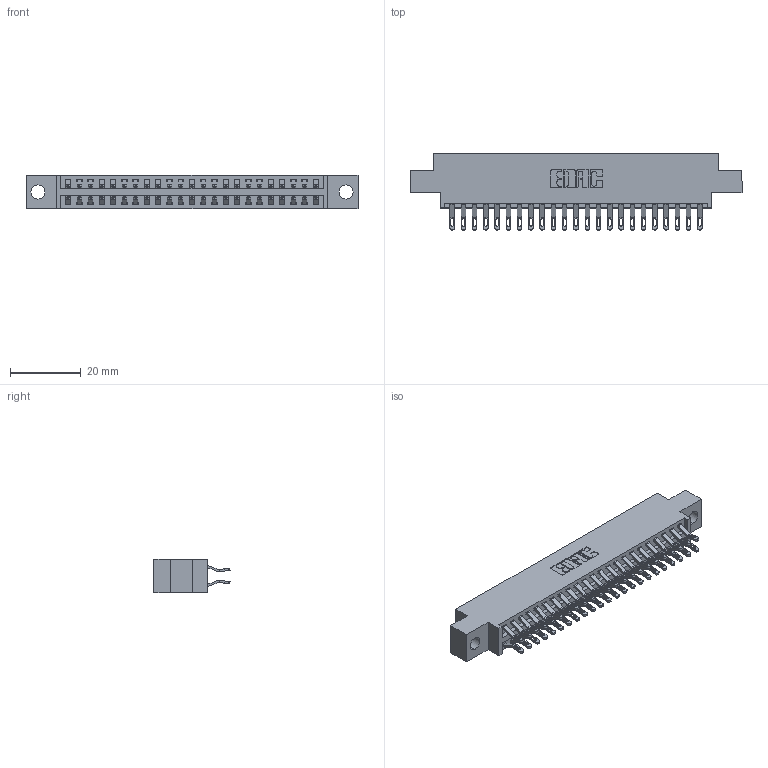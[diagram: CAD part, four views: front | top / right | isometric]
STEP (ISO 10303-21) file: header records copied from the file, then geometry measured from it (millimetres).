
FILE_DESCRIPTION (( 'STEP AP203' ), '1' );
FILE_NAME ('396-046-555-804.STEP', '2018-09-07T09:04:24', ( '' ), ( '' ), 'SwSTEP 2.0', 'SolidWorks 2016', '' );
FILE_SCHEMA (( 'CONFIG_CONTROL_DESIGN' ));
Length unit declared in the file: inch
Products named in the file (3): 346 Part_0.170 Offset - 0.156 Dia-TH; 345-292-001_555 Tail; 396-046-555-804
Assembly tree (47 placements, depth 2):
  396-046-555-804
    346 Part_0.170 Offset - 0.156 Dia-TH
    345-292-001_555 Tail  x46
Bounding box: 93.6 x 21.46 x 9.4 mm (x, y, z)
Volume: 8870.5 mm3; surface area: 12363 mm2
Topology: 47 solids, 47 shells, 2794 faces, 8759 edges, 5838 vertices
Faces by surface type: plane 1598, cylinder 1196
Entity records: 18029 total; most frequent: CARTESIAN_POINT 3034, ORIENTED_EDGE 2938, DIRECTION 2693, EDGE_CURVE 1469, VECTOR 1225, LINE 1225, VERTEX_POINT 978, AXIS2_PLACEMENT_3D 734
